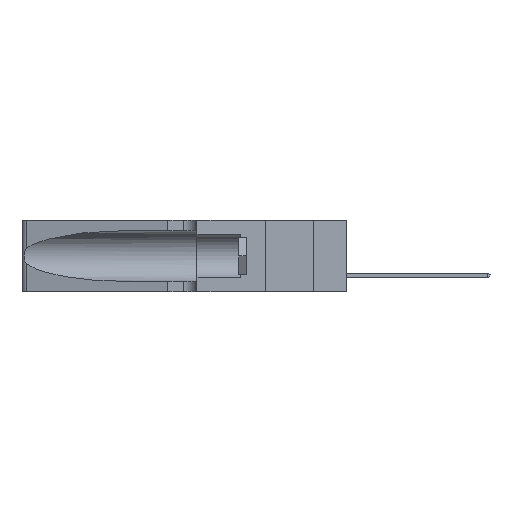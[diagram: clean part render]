
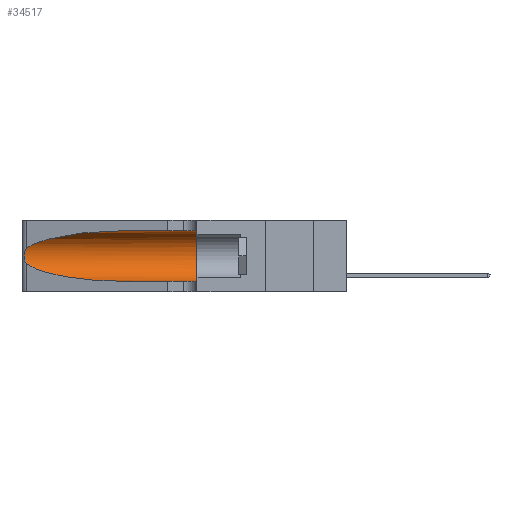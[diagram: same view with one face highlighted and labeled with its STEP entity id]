
A CAD part, left-side view. The second image highlights one B-rep face of the part: STEP entity #34517.
In plain terms, the highlighted cylindrical face has radius 3.308 mm (diameter 6.617 mm), a partial arc.
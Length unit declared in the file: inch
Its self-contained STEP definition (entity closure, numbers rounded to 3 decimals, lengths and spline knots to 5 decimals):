
#71 = CARTESIAN_POINT ( 'NONE',  ( 0.25487, 1.22718, 0.22369 ) ) ;
#503 = CARTESIAN_POINT ( 'NONE',  ( 0.25854, 1.2359, 0.20912 ) ) ;
#1085 = CARTESIAN_POINT ( 'NONE',  ( 0.25487, 1.22718, 0.14631 ) ) ;
#1770 = EDGE_CURVE ( 'NONE', #18302, #41267, #33093, .T. ) ;
#2151 = CARTESIAN_POINT ( 'NONE',  ( 0.1305, 1.61858, 0.31525 ) ) ;
#2410 = AXIS2_PLACEMENT_3D ( 'NONE', #28725, #28116, #31986 ) ;
#2591 = CARTESIAN_POINT ( 'NONE',  ( 0.2373, 1.15595, 0.08982 ) ) ;
#3111 = CARTESIAN_POINT ( 'NONE',  ( 0.25487, 1.22718, 0.14631 ) ) ;
#3624 = CARTESIAN_POINT ( 'NONE',  ( 0.26075, 1.23896, 0.178 ) ) ;
#4039 = CARTESIAN_POINT ( 'NONE',  ( 0.26017, 1.23833, 0.17102 ) ) ;
#5760 = CARTESIAN_POINT ( 'NONE',  ( 0.25555, 1.22994, 0.2215 ) ) ;
#7052 =( BOUNDED_CURVE ( )  B_SPLINE_CURVE ( 3, ( #36857, #2591, #9561, #43209 ),
 .UNSPECIFIED., .F., .F. ) 
 B_SPLINE_CURVE_WITH_KNOTS ( ( 4, 4 ),
 ( 3.44316, 4.71239 ),
 .UNSPECIFIED. ) 
 CURVE ( )  GEOMETRIC_REPRESENTATION_ITEM ( )  RATIONAL_B_SPLINE_CURVE ( ( 1., 0.87, 0.87, 1. ) ) 
 REPRESENTATION_ITEM ( '' )  );
#7519 = CARTESIAN_POINT ( 'NONE',  ( 0.26018, 1.23835, 0.19895 ) ) ;
#7663 = CARTESIAN_POINT ( 'NONE',  ( 0.25789, 1.23486, 0.15765 ) ) ;
#7861 = CARTESIAN_POINT ( 'NONE',  ( 0.1305, 0.72297, 0.31525 ) ) ;
#7871 = ORIENTED_EDGE ( 'NONE', *, *, #30177, .F. ) ;
#8773 = LINE ( 'NONE', #42015, #36175 ) ;
#9011 = CARTESIAN_POINT ( 'NONE',  ( 0.1305, 0.35, 0.31525 ) ) ;
#9104 = CARTESIAN_POINT ( 'NONE',  ( 0.1305, 0.72297, 0.05475 ) ) ;
#9253 = VERTEX_POINT ( 'NONE', #9104 ) ;
#9561 = CARTESIAN_POINT ( 'NONE',  ( 0.18966, 0.96281, 0.05475 ) ) ;
#11025 = CARTESIAN_POINT ( 'NONE',  ( 0.25639, 1.23186, 0.15144 ) ) ;
#11245 = CARTESIAN_POINT ( 'NONE',  ( 0.18966, 0.96281, 0.31525 ) ) ;
#12078 = CARTESIAN_POINT ( 'NONE',  ( 0.1305, 0.35, 0.05475 ) ) ;
#12782 = DIRECTION ( 'NONE',  ( 0., -1., 0. ) ) ;
#13738 = AXIS2_PLACEMENT_3D ( 'NONE', #33910, #34182, #30932 ) ;
#15800 = EDGE_LOOP ( 'NONE', ( #37412, #17548, #17358, #23076, #7871, #34355 ) ) ;
#17286 = CARTESIAN_POINT ( 'NONE',  ( 0.2373, 1.15595, 0.28018 ) ) ;
#17358 = ORIENTED_EDGE ( 'NONE', *, *, #19074, .T. ) ;
#17391 = EDGE_CURVE ( 'NONE', #9253, #26701, #8773, .T. ) ;
#17548 = ORIENTED_EDGE ( 'NONE', *, *, #1770, .T. ) ;
#17758 = CYLINDRICAL_SURFACE ( 'NONE', #2410, 0.13025 ) ;
#18302 = VERTEX_POINT ( 'NONE', #28337 ) ;
#18723 =( BOUNDED_CURVE ( )  B_SPLINE_CURVE ( 3, ( #7861, #11245, #17286, #20699 ),
 .UNSPECIFIED., .F., .F. ) 
 B_SPLINE_CURVE_WITH_KNOTS ( ( 4, 4 ),
 ( 1.5708, 2.84003 ),
 .UNSPECIFIED. ) 
 CURVE ( )  GEOMETRIC_REPRESENTATION_ITEM ( )  RATIONAL_B_SPLINE_CURVE ( ( 1., 0.87, 0.87, 1. ) ) 
 REPRESENTATION_ITEM ( '' )  );
#19074 = EDGE_CURVE ( 'NONE', #41267, #9253, #7052, .T. ) ;
#19337 = EDGE_CURVE ( 'NONE', #21103, #43015, #34974, .T. ) ;
#20699 = CARTESIAN_POINT ( 'NONE',  ( 0.25487, 1.22718, 0.22369 ) ) ;
#21103 = VERTEX_POINT ( 'NONE', #34074 ) ;
#21183 = DIRECTION ( 'NONE',  ( 0., -1., 0. ) ) ;
#23076 = ORIENTED_EDGE ( 'NONE', *, *, #17391, .T. ) ;
#23399 = CARTESIAN_POINT ( 'NONE',  ( 0.25639, 1.23184, 0.21858 ) ) ;
#23633 = EDGE_CURVE ( 'NONE', #21103, #18302, #18723, .T. ) ;
#24158 = CARTESIAN_POINT ( 'NONE',  ( 0.26075, 1.23896, 0.19203 ) ) ;
#26040 = VECTOR ( 'NONE', #12782, 39.37008 ) ;
#26701 = VERTEX_POINT ( 'NONE', #12078 ) ;
#27857 = CARTESIAN_POINT ( 'NONE',  ( 0.25856, 1.23593, 0.16098 ) ) ;
#28116 = DIRECTION ( 'NONE',  ( 0., -1., 0. ) ) ;
#28337 = CARTESIAN_POINT ( 'NONE',  ( 0.25487, 1.22718, 0.22369 ) ) ;
#28725 = CARTESIAN_POINT ( 'NONE',  ( 0.1305, 1.61858, 0.185 ) ) ;
#30177 = EDGE_CURVE ( 'NONE', #43015, #26701, #36366, .T. ) ;
#30932 = DIRECTION ( 'NONE',  ( 0., 0., 1. ) ) ;
#31986 = DIRECTION ( 'NONE',  ( 0., 0., -1. ) ) ;
#33093 = B_SPLINE_CURVE_WITH_KNOTS ( 'NONE', 3,
 ( #71, #5760, #23399, #34534, #503, #7519, #24158, #3624, #4039, #27857, #7663, #11025, #35107, #1085 ),
 .UNSPECIFIED., .F., .F.,
 ( 4, 2, 2, 2, 2, 2, 4 ),
 ( 0., 0.00027, 0.00053, 0.00107, 0.0016, 0.00187, 0.00214 ),
 .UNSPECIFIED. ) ;
#33910 = CARTESIAN_POINT ( 'NONE',  ( 0.1305, 0.35, 0.185 ) ) ;
#34074 = CARTESIAN_POINT ( 'NONE',  ( 0.1305, 0.72297, 0.31525 ) ) ;
#34182 = DIRECTION ( 'NONE',  ( 0., 1., 0. ) ) ;
#34355 = ORIENTED_EDGE ( 'NONE', *, *, #19337, .F. ) ;
#34517 = ADVANCED_FACE ( 'NONE', ( #40005 ), #17758, .F. ) ;
#34534 = CARTESIAN_POINT ( 'NONE',  ( 0.25787, 1.23484, 0.2124 ) ) ;
#34974 = LINE ( 'NONE', #2151, #26040 ) ;
#35107 = CARTESIAN_POINT ( 'NONE',  ( 0.25555, 1.22993, 0.14849 ) ) ;
#36175 = VECTOR ( 'NONE', #21183, 39.37008 ) ;
#36366 = CIRCLE ( 'NONE', #13738, 0.13025 ) ;
#36857 = CARTESIAN_POINT ( 'NONE',  ( 0.25487, 1.22718, 0.14631 ) ) ;
#37412 = ORIENTED_EDGE ( 'NONE', *, *, #23633, .T. ) ;
#40005 = FACE_OUTER_BOUND ( 'NONE', #15800, .T. ) ;
#41267 = VERTEX_POINT ( 'NONE', #3111 ) ;
#42015 = CARTESIAN_POINT ( 'NONE',  ( 0.1305, 1.61858, 0.05475 ) ) ;
#43015 = VERTEX_POINT ( 'NONE', #9011 ) ;
#43209 = CARTESIAN_POINT ( 'NONE',  ( 0.1305, 0.72297, 0.05475 ) ) ;
